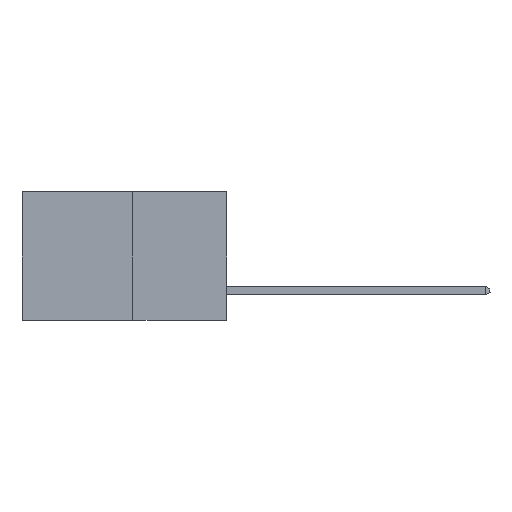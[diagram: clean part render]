
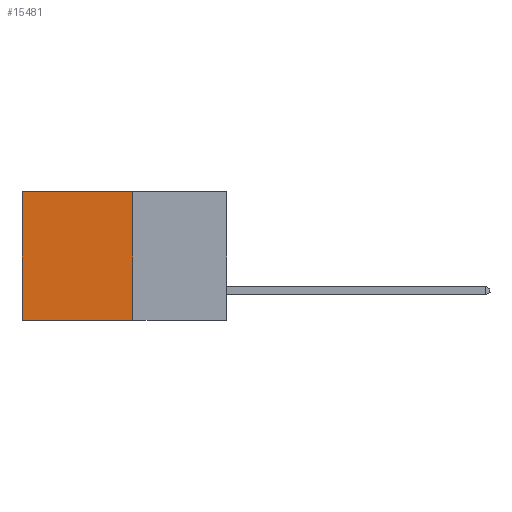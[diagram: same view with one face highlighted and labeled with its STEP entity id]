
A CAD part, left-side view. The second image highlights one B-rep face of the part: STEP entity #15481.
In plain terms, the highlighted planar face has unit normal (-1, 0, 0).
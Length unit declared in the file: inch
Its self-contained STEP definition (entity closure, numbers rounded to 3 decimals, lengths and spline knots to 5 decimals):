
#100 = LINE ( 'NONE', #7324, #20800 ) ;
#980 = VERTEX_POINT ( 'NONE', #11429 ) ;
#1048 = VECTOR ( 'NONE', #17745, 39.37008 ) ;
#1208 = CARTESIAN_POINT ( 'NONE',  ( 0.277, 0.27, -0.37 ) ) ;
#1794 = DIRECTION ( 'NONE',  ( 0., 0., -1. ) ) ;
#2497 = EDGE_CURVE ( 'NONE', #980, #6888, #19495, .T. ) ;
#5933 = LINE ( 'NONE', #1208, #1048 ) ;
#6099 = CARTESIAN_POINT ( 'NONE',  ( 0.277, 0.27, -0.37 ) ) ;
#6837 = FACE_OUTER_BOUND ( 'NONE', #13504, .T. ) ;
#6888 = VERTEX_POINT ( 'NONE', #24472 ) ;
#7324 = CARTESIAN_POINT ( 'NONE',  ( 0.277, 0.27, -0.37 ) ) ;
#7813 = VECTOR ( 'NONE', #1794, 39.37008 ) ;
#8142 = DIRECTION ( 'NONE',  ( 0., 0., -1. ) ) ;
#8452 = AXIS2_PLACEMENT_3D ( 'NONE', #6099, #20508, #8142 ) ;
#8651 = CARTESIAN_POINT ( 'NONE',  ( 0.277, 0.27, 0. ) ) ;
#10849 = CARTESIAN_POINT ( 'NONE',  ( 0.277, 0.59, -0.37 ) ) ;
#11429 = CARTESIAN_POINT ( 'NONE',  ( 0.277, 0.59, 0. ) ) ;
#11431 = VERTEX_POINT ( 'NONE', #18315 ) ;
#11604 = ORIENTED_EDGE ( 'NONE', *, *, #22199, .T. ) ;
#13433 = DIRECTION ( 'NONE',  ( 0., 1., 0. ) ) ;
#13504 = EDGE_LOOP ( 'NONE', ( #19299, #13892, #14477, #11604 ) ) ;
#13876 = EDGE_CURVE ( 'NONE', #11431, #6888, #100, .T. ) ;
#13892 = ORIENTED_EDGE ( 'NONE', *, *, #13876, .F. ) ;
#14248 = PLANE ( 'NONE',  #8452 ) ;
#14477 = ORIENTED_EDGE ( 'NONE', *, *, #26598, .F. ) ;
#15481 = ADVANCED_FACE ( 'NONE', ( #6837 ), #14248, .F. ) ;
#17745 = DIRECTION ( 'NONE',  ( 0., 0., -1. ) ) ;
#18315 = CARTESIAN_POINT ( 'NONE',  ( 0.277, 0.27, -0.37 ) ) ;
#19299 = ORIENTED_EDGE ( 'NONE', *, *, #2497, .T. ) ;
#19495 = LINE ( 'NONE', #10849, #7813 ) ;
#20508 = DIRECTION ( 'NONE',  ( 1., 0., 0. ) ) ;
#20800 = VECTOR ( 'NONE', #13433, 39.37008 ) ;
#22079 = CARTESIAN_POINT ( 'NONE',  ( 0.277, 0.27, 0. ) ) ;
#22199 = EDGE_CURVE ( 'NONE', #26018, #980, #24491, .T. ) ;
#23094 = DIRECTION ( 'NONE',  ( 0., 1., 0. ) ) ;
#23833 = VECTOR ( 'NONE', #23094, 39.37008 ) ;
#24472 = CARTESIAN_POINT ( 'NONE',  ( 0.277, 0.59, -0.37 ) ) ;
#24491 = LINE ( 'NONE', #8651, #23833 ) ;
#26018 = VERTEX_POINT ( 'NONE', #22079 ) ;
#26598 = EDGE_CURVE ( 'NONE', #26018, #11431, #5933, .T. ) ;
